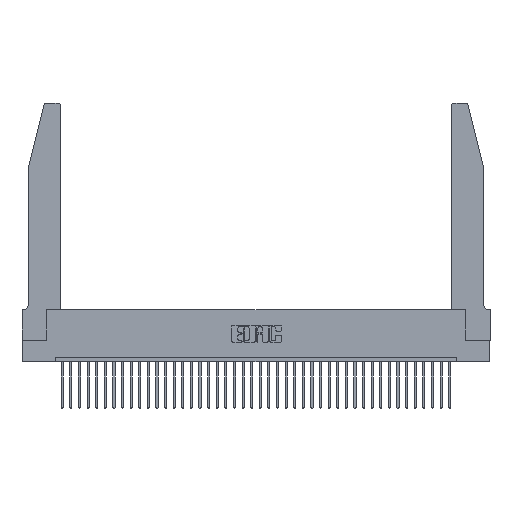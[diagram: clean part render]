
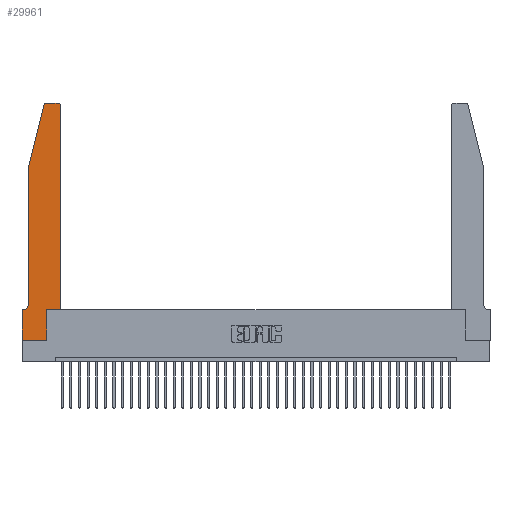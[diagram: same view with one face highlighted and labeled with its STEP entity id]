
A CAD part, top view. The second image highlights one B-rep face of the part: STEP entity #29961.
In plain terms, the highlighted planar face has unit normal (0, 0, 1).
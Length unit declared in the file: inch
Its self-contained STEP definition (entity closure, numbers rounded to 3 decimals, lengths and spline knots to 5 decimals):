
#1694 = VECTOR ( 'NONE', #22492, 39.37008 ) ;
#2114 = CARTESIAN_POINT ( 'NONE',  ( 0.2605, 2.75, 0.37 ) ) ;
#2240 = VERTEX_POINT ( 'NONE', #7691 ) ;
#2461 = EDGE_LOOP ( 'NONE', ( #31814, #15840, #2588, #11855, #13278, #19396, #2702, #5443, #18628, #10839, #33723, #19307 ) ) ;
#2588 = ORIENTED_EDGE ( 'NONE', *, *, #19491, .T. ) ;
#2702 = ORIENTED_EDGE ( 'NONE', *, *, #4597, .T. ) ;
#3270 = LINE ( 'NONE', #4509, #29485 ) ;
#4151 = AXIS2_PLACEMENT_3D ( 'NONE', #23614, #17727, #20734 ) ;
#4509 = CARTESIAN_POINT ( 'NONE',  ( 0., 0., 0.37 ) ) ;
#4597 = EDGE_CURVE ( 'NONE', #11636, #2240, #3270, .T. ) ;
#4978 = VECTOR ( 'NONE', #37812, 39.37008 ) ;
#5204 = CARTESIAN_POINT ( 'NONE',  ( 0.284, 2.75, 0.37 ) ) ;
#5443 = ORIENTED_EDGE ( 'NONE', *, *, #30550, .T. ) ;
#6216 = CARTESIAN_POINT ( 'NONE',  ( 0.0755, 2., 0.37 ) ) ;
#7015 = CARTESIAN_POINT ( 'NONE',  ( 0.0755, 2., 0.37 ) ) ;
#7681 = DIRECTION ( 'NONE',  ( 0., -1., 0. ) ) ;
#7691 = CARTESIAN_POINT ( 'NONE',  ( 0., 0., 0.37 ) ) ;
#8131 = CARTESIAN_POINT ( 'NONE',  ( 0.0055, 0.42, 0.37 ) ) ;
#8203 = CARTESIAN_POINT ( 'NONE',  ( 0.0755, 2., 0.37 ) ) ;
#9281 = LINE ( 'NONE', #35061, #37882 ) ;
#9738 = CIRCLE ( 'NONE', #10568, 0.03 ) ;
#9874 = CARTESIAN_POINT ( 'NONE',  ( 0.25487, 2.72718, 0.37 ) ) ;
#10453 = DIRECTION ( 'NONE',  ( -0.239, -0.971, 0. ) ) ;
#10568 = AXIS2_PLACEMENT_3D ( 'NONE', #16857, #17115, #28764 ) ;
#10722 = CARTESIAN_POINT ( 'NONE',  ( 0.0755, 0.35, 0.37 ) ) ;
#10839 = ORIENTED_EDGE ( 'NONE', *, *, #23063, .T. ) ;
#10851 = PLANE ( 'NONE',  #35094 ) ;
#10977 = CARTESIAN_POINT ( 'NONE',  ( 0.2865, 0.35, 0.37 ) ) ;
#11379 = CIRCLE ( 'NONE', #4151, 0.03 ) ;
#11387 = VERTEX_POINT ( 'NONE', #18623 ) ;
#11636 = VERTEX_POINT ( 'NONE', #32783 ) ;
#11855 = ORIENTED_EDGE ( 'NONE', *, *, #13365, .T. ) ;
#11960 = LINE ( 'NONE', #19942, #36781 ) ;
#12807 = CARTESIAN_POINT ( 'NONE',  ( 0.4505, 0.35, 0.37 ) ) ;
#13128 = CARTESIAN_POINT ( 'NONE',  ( 0.4205, 2.75, 0.37 ) ) ;
#13278 = ORIENTED_EDGE ( 'NONE', *, *, #18033, .T. ) ;
#13365 = EDGE_CURVE ( 'NONE', #32894, #11387, #19742, .T. ) ;
#13751 = VECTOR ( 'NONE', #10453, 39.37008 ) ;
#14254 = DIRECTION ( 'NONE',  ( 0., 0., 1. ) ) ;
#14505 = AXIS2_PLACEMENT_3D ( 'NONE', #8131, #38000, #32541 ) ;
#14991 = EDGE_CURVE ( 'NONE', #34541, #33231, #9738, .T. ) ;
#15071 = VERTEX_POINT ( 'NONE', #21795 ) ;
#15426 = VERTEX_POINT ( 'NONE', #33373 ) ;
#15840 = ORIENTED_EDGE ( 'NONE', *, *, #14991, .T. ) ;
#16857 = CARTESIAN_POINT ( 'NONE',  ( 0.284, 2.72, 0.37 ) ) ;
#17115 = DIRECTION ( 'NONE',  ( 0., 0., 1. ) ) ;
#17533 = LINE ( 'NONE', #7015, #13751 ) ;
#17653 = DIRECTION ( 'NONE',  ( 0., 1., 0. ) ) ;
#17727 = DIRECTION ( 'NONE',  ( 0., 0., 1. ) ) ;
#17991 = EDGE_CURVE ( 'NONE', #15426, #19866, #11960, .T. ) ;
#18033 = EDGE_CURVE ( 'NONE', #11387, #29987, #19452, .T. ) ;
#18623 = CARTESIAN_POINT ( 'NONE',  ( 0.0755, 0.42, 0.37 ) ) ;
#18628 = ORIENTED_EDGE ( 'NONE', *, *, #17991, .T. ) ;
#19305 = EDGE_CURVE ( 'NONE', #15071, #20932, #11379, .T. ) ;
#19307 = ORIENTED_EDGE ( 'NONE', *, *, #19305, .T. ) ;
#19396 = ORIENTED_EDGE ( 'NONE', *, *, #32892, .T. ) ;
#19452 = CIRCLE ( 'NONE', #14505, 0.07 ) ;
#19491 = EDGE_CURVE ( 'NONE', #33231, #32894, #17533, .T. ) ;
#19742 = LINE ( 'NONE', #6216, #35685 ) ;
#19745 = DIRECTION ( 'NONE',  ( 1., 0., 0. ) ) ;
#19866 = VERTEX_POINT ( 'NONE', #10977 ) ;
#19877 = CARTESIAN_POINT ( 'NONE',  ( 0.0055, 0.35, 0.37 ) ) ;
#19942 = CARTESIAN_POINT ( 'NONE',  ( 0.2865, 0.35, 0.37 ) ) ;
#20714 = VERTEX_POINT ( 'NONE', #12807 ) ;
#20734 = DIRECTION ( 'NONE',  ( 1., 0., 0. ) ) ;
#20932 = VERTEX_POINT ( 'NONE', #13128 ) ;
#21795 = CARTESIAN_POINT ( 'NONE',  ( 0.4505, 2.72, 0.37 ) ) ;
#22492 = DIRECTION ( 'NONE',  ( 1., 0., 0. ) ) ;
#22502 = EDGE_CURVE ( 'NONE', #20714, #15071, #9281, .T. ) ;
#23063 = EDGE_CURVE ( 'NONE', #19866, #20714, #27495, .T. ) ;
#23288 = CARTESIAN_POINT ( 'NONE',  ( 0., 0.35, 0.37 ) ) ;
#23614 = CARTESIAN_POINT ( 'NONE',  ( 0.4205, 2.72, 0.37 ) ) ;
#25759 = VECTOR ( 'NONE', #35575, 39.37008 ) ;
#27495 = LINE ( 'NONE', #37376, #1694 ) ;
#27971 = LINE ( 'NONE', #10722, #4978 ) ;
#28764 = DIRECTION ( 'NONE',  ( 1., 0., 0. ) ) ;
#29485 = VECTOR ( 'NONE', #7681, 39.37008 ) ;
#29961 = ADVANCED_FACE ( 'NONE', ( #35210 ), #10851, .T. ) ;
#29987 = VERTEX_POINT ( 'NONE', #19877 ) ;
#30390 = EDGE_CURVE ( 'NONE', #20932, #34541, #38462, .T. ) ;
#30550 = EDGE_CURVE ( 'NONE', #2240, #15426, #31430, .T. ) ;
#31430 = LINE ( 'NONE', #38680, #25759 ) ;
#31629 = DIRECTION ( 'NONE',  ( 0., 1., 0. ) ) ;
#31814 = ORIENTED_EDGE ( 'NONE', *, *, #30390, .T. ) ;
#32541 = DIRECTION ( 'NONE',  ( -1., 0., 0. ) ) ;
#32783 = CARTESIAN_POINT ( 'NONE',  ( 0., 0.35, 0.37 ) ) ;
#32892 = EDGE_CURVE ( 'NONE', #29987, #11636, #27971, .T. ) ;
#32894 = VERTEX_POINT ( 'NONE', #8203 ) ;
#33231 = VERTEX_POINT ( 'NONE', #9874 ) ;
#33373 = CARTESIAN_POINT ( 'NONE',  ( 0.2865, 0., 0.37 ) ) ;
#33723 = ORIENTED_EDGE ( 'NONE', *, *, #22502, .T. ) ;
#34541 = VERTEX_POINT ( 'NONE', #5204 ) ;
#34924 = DIRECTION ( 'NONE',  ( -1., 0., 0. ) ) ;
#35061 = CARTESIAN_POINT ( 'NONE',  ( 0.4505, 0.35, 0.37 ) ) ;
#35094 = AXIS2_PLACEMENT_3D ( 'NONE', #23288, #14254, #19745 ) ;
#35210 = FACE_OUTER_BOUND ( 'NONE', #2461, .T. ) ;
#35575 = DIRECTION ( 'NONE',  ( 1., 0., 0. ) ) ;
#35658 = VECTOR ( 'NONE', #34924, 39.37008 ) ;
#35685 = VECTOR ( 'NONE', #35811, 39.37008 ) ;
#35811 = DIRECTION ( 'NONE',  ( 0., -1., 0. ) ) ;
#36781 = VECTOR ( 'NONE', #31629, 39.37008 ) ;
#37376 = CARTESIAN_POINT ( 'NONE',  ( 0.4505, 0.35, 0.37 ) ) ;
#37812 = DIRECTION ( 'NONE',  ( -1., 0., 0. ) ) ;
#37882 = VECTOR ( 'NONE', #17653, 39.37008 ) ;
#38000 = DIRECTION ( 'NONE',  ( 0., 0., -1. ) ) ;
#38462 = LINE ( 'NONE', #2114, #35658 ) ;
#38680 = CARTESIAN_POINT ( 'NONE',  ( 0., 0., 0.37 ) ) ;
